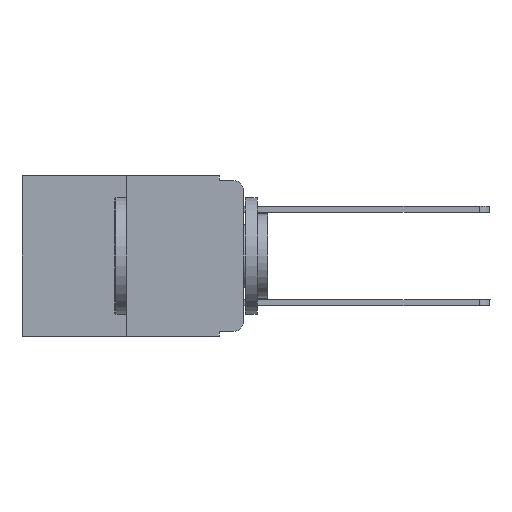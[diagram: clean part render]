
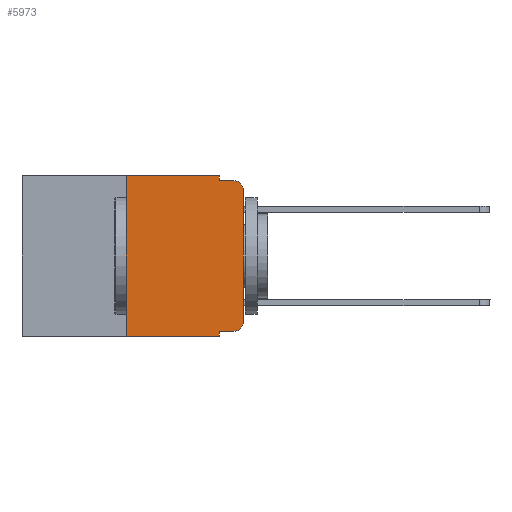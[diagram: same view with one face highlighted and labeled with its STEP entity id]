
A CAD part, left-side view. The second image highlights one B-rep face of the part: STEP entity #5973.
In plain terms, the highlighted planar face has unit normal (-1, 0, 0).
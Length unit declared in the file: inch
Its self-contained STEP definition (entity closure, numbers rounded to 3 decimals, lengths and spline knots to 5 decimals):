
#25 = ORIENTED_EDGE ( 'NONE', *, *, #10498, .F. ) ;
#42 = VECTOR ( 'NONE', #6534, 39.37008 ) ;
#193 = DIRECTION ( 'NONE',  ( 0., 0., -1. ) ) ;
#265 = VERTEX_POINT ( 'NONE', #1996 ) ;
#305 = DIRECTION ( 'NONE',  ( 0., 0., 1. ) ) ;
#407 = VECTOR ( 'NONE', #10155, 39.37008 ) ;
#469 = VERTEX_POINT ( 'NONE', #5744 ) ;
#580 = EDGE_CURVE ( 'NONE', #10437, #4559, #3384, .T. ) ;
#941 = DIRECTION ( 'NONE',  ( 0., 0., -1. ) ) ;
#1177 = VECTOR ( 'NONE', #7493, 39.37008 ) ;
#1201 = EDGE_CURVE ( 'NONE', #265, #4170, #7652, .T. ) ;
#1299 = DIRECTION ( 'NONE',  ( 1., 0., 0. ) ) ;
#1504 = VERTEX_POINT ( 'NONE', #8459 ) ;
#1696 = CARTESIAN_POINT ( 'NONE',  ( 0., 0.051, -0.01 ) ) ;
#1912 = CIRCLE ( 'NONE', #7809, 0.02 ) ;
#1933 = LINE ( 'NONE', #12308, #11139 ) ;
#1947 = DIRECTION ( 'NONE',  ( 0., 0., -1. ) ) ;
#1996 = CARTESIAN_POINT ( 'NONE',  ( 0., 0.25, -0.343 ) ) ;
#2077 = VECTOR ( 'NONE', #1947, 39.37008 ) ;
#2312 = ORIENTED_EDGE ( 'NONE', *, *, #580, .T. ) ;
#2337 = VECTOR ( 'NONE', #193, 39.37008 ) ;
#2563 = ORIENTED_EDGE ( 'NONE', *, *, #4190, .T. ) ;
#2617 = VECTOR ( 'NONE', #305, 39.37008 ) ;
#2814 = LINE ( 'NONE', #5882, #2077 ) ;
#2964 = LINE ( 'NONE', #5458, #407 ) ;
#3068 = CARTESIAN_POINT ( 'NONE',  ( 0., 0.051, 0. ) ) ;
#3282 = ORIENTED_EDGE ( 'NONE', *, *, #11689, .F. ) ;
#3384 = LINE ( 'NONE', #4931, #5292 ) ;
#3515 = CARTESIAN_POINT ( 'NONE',  ( 0., 0.02, -0.333 ) ) ;
#3833 = ORIENTED_EDGE ( 'NONE', *, *, #6343, .F. ) ;
#4116 = AXIS2_PLACEMENT_3D ( 'NONE', #5465, #8291, #7443 ) ;
#4133 = LINE ( 'NONE', #9054, #1177 ) ;
#4170 = VERTEX_POINT ( 'NONE', #12095 ) ;
#4190 = EDGE_CURVE ( 'NONE', #265, #4295, #4133, .T. ) ;
#4295 = VERTEX_POINT ( 'NONE', #7617 ) ;
#4321 = VERTEX_POINT ( 'NONE', #10505 ) ;
#4559 = VERTEX_POINT ( 'NONE', #3515 ) ;
#4931 = CARTESIAN_POINT ( 'NONE',  ( 0., 0.051, -0.333 ) ) ;
#5197 = DIRECTION ( 'NONE',  ( 0., 0., -1. ) ) ;
#5292 = VECTOR ( 'NONE', #9557, 39.37008 ) ;
#5420 = CIRCLE ( 'NONE', #4116, 0.02 ) ;
#5458 = CARTESIAN_POINT ( 'NONE',  ( 0., 0.473, 0. ) ) ;
#5465 = CARTESIAN_POINT ( 'NONE',  ( 0., 0.02, -0.313 ) ) ;
#5594 = VERTEX_POINT ( 'NONE', #9921 ) ;
#5744 = CARTESIAN_POINT ( 'NONE',  ( 0., 0.051, -0.01 ) ) ;
#5775 = AXIS2_PLACEMENT_3D ( 'NONE', #6978, #1299, #5197 ) ;
#5882 = CARTESIAN_POINT ( 'NONE',  ( 0., 0.051, 0. ) ) ;
#5973 = ADVANCED_FACE ( 'NONE', ( #11828 ), #11678, .F. ) ;
#6262 = EDGE_CURVE ( 'NONE', #4559, #1504, #5420, .T. ) ;
#6343 = EDGE_CURVE ( 'NONE', #469, #5594, #10491, .T. ) ;
#6527 = DIRECTION ( 'NONE',  ( -1., 0., 0. ) ) ;
#6534 = DIRECTION ( 'NONE',  ( 0., -1., 0. ) ) ;
#6651 = ORIENTED_EDGE ( 'NONE', *, *, #9335, .T. ) ;
#6786 = DIRECTION ( 'NONE',  ( 0., 0., 1. ) ) ;
#6978 = CARTESIAN_POINT ( 'NONE',  ( 0., 0.473, 0. ) ) ;
#7108 = ORIENTED_EDGE ( 'NONE', *, *, #10668, .F. ) ;
#7125 = CARTESIAN_POINT ( 'NONE',  ( 0., 0.25, 0. ) ) ;
#7443 = DIRECTION ( 'NONE',  ( 0., 0., -1. ) ) ;
#7493 = DIRECTION ( 'NONE',  ( 0., -1., 0. ) ) ;
#7617 = CARTESIAN_POINT ( 'NONE',  ( 0., 0.051, -0.343 ) ) ;
#7652 = LINE ( 'NONE', #7125, #2617 ) ;
#7803 = ORIENTED_EDGE ( 'NONE', *, *, #6262, .T. ) ;
#7809 = AXIS2_PLACEMENT_3D ( 'NONE', #11360, #6527, #941 ) ;
#7915 = CARTESIAN_POINT ( 'NONE',  ( 0., 0.051, 0. ) ) ;
#8291 = DIRECTION ( 'NONE',  ( -1., 0., 0. ) ) ;
#8353 = VERTEX_POINT ( 'NONE', #7915 ) ;
#8459 = CARTESIAN_POINT ( 'NONE',  ( 0., 0., -0.313 ) ) ;
#9054 = CARTESIAN_POINT ( 'NONE',  ( 0., 0.473, -0.343 ) ) ;
#9283 = ORIENTED_EDGE ( 'NONE', *, *, #10787, .T. ) ;
#9335 = EDGE_CURVE ( 'NONE', #1504, #4321, #1933, .T. ) ;
#9557 = DIRECTION ( 'NONE',  ( 0., -1., 0. ) ) ;
#9921 = CARTESIAN_POINT ( 'NONE',  ( 0., 0.02, -0.01 ) ) ;
#10108 = ORIENTED_EDGE ( 'NONE', *, *, #1201, .F. ) ;
#10155 = DIRECTION ( 'NONE',  ( 0., -1., 0. ) ) ;
#10437 = VERTEX_POINT ( 'NONE', #11624 ) ;
#10472 = EDGE_LOOP ( 'NONE', ( #6651, #9283, #3833, #25, #7108, #10108, #2563, #3282, #2312, #7803 ) ) ;
#10491 = LINE ( 'NONE', #1696, #42 ) ;
#10498 = EDGE_CURVE ( 'NONE', #8353, #469, #2814, .T. ) ;
#10505 = CARTESIAN_POINT ( 'NONE',  ( 0., 0., -0.03 ) ) ;
#10668 = EDGE_CURVE ( 'NONE', #4170, #8353, #2964, .T. ) ;
#10787 = EDGE_CURVE ( 'NONE', #4321, #5594, #1912, .T. ) ;
#11139 = VECTOR ( 'NONE', #6786, 39.37008 ) ;
#11248 = LINE ( 'NONE', #3068, #2337 ) ;
#11360 = CARTESIAN_POINT ( 'NONE',  ( 0., 0.02, -0.03 ) ) ;
#11624 = CARTESIAN_POINT ( 'NONE',  ( 0., 0.051, -0.333 ) ) ;
#11678 = PLANE ( 'NONE',  #5775 ) ;
#11689 = EDGE_CURVE ( 'NONE', #10437, #4295, #11248, .T. ) ;
#11828 = FACE_OUTER_BOUND ( 'NONE', #10472, .T. ) ;
#12095 = CARTESIAN_POINT ( 'NONE',  ( 0., 0.25, 0. ) ) ;
#12308 = CARTESIAN_POINT ( 'NONE',  ( 0., 0., 0. ) ) ;
